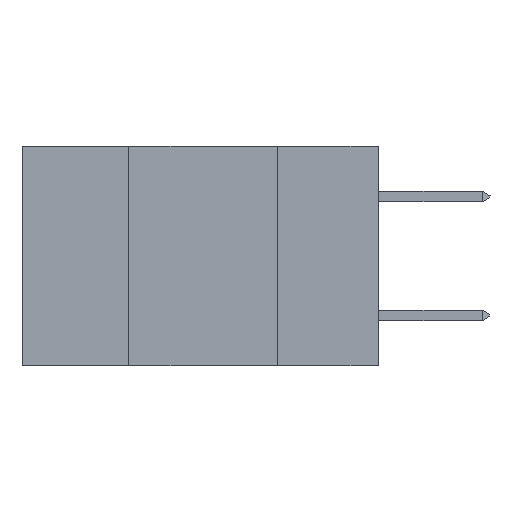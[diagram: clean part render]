
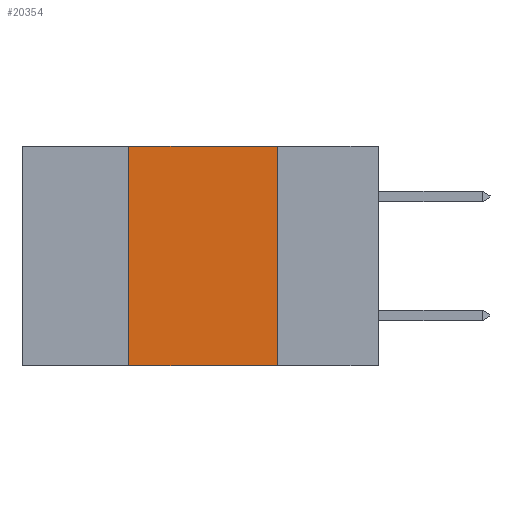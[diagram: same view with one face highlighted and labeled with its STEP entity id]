
A CAD part, left-side view. The second image highlights one B-rep face of the part: STEP entity #20354.
In plain terms, the highlighted planar face has unit normal (-1, 0, 0).
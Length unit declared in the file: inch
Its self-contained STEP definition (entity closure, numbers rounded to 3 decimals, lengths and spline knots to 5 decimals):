
#238 = LINE ( 'NONE', #11202, #19931 ) ;
#572 = VERTEX_POINT ( 'NONE', #11583 ) ;
#872 = EDGE_CURVE ( 'NONE', #572, #17587, #2116, .T. ) ;
#2116 = LINE ( 'NONE', #15072, #17756 ) ;
#3079 = DIRECTION ( 'NONE',  ( 0., 0., -1. ) ) ;
#4374 = DIRECTION ( 'NONE',  ( 0., -1., 0. ) ) ;
#5591 = CARTESIAN_POINT ( 'NONE',  ( 0., 0.6, 0. ) ) ;
#8666 = DIRECTION ( 'NONE',  ( 0., 0., -1. ) ) ;
#9419 = FACE_OUTER_BOUND ( 'NONE', #26075, .T. ) ;
#10312 = CARTESIAN_POINT ( 'NONE',  ( 0., 0.42, -0.37 ) ) ;
#10592 = CARTESIAN_POINT ( 'NONE',  ( 0., 0.17, 0. ) ) ;
#11069 = EDGE_CURVE ( 'NONE', #572, #26701, #14545, .T. ) ;
#11202 = CARTESIAN_POINT ( 'NONE',  ( 0., 0.17, -0.37 ) ) ;
#11583 = CARTESIAN_POINT ( 'NONE',  ( 0., 0.42, -0.37 ) ) ;
#12337 = ORIENTED_EDGE ( 'NONE', *, *, #26849, .F. ) ;
#13105 = VECTOR ( 'NONE', #18578, 39.37008 ) ;
#14545 = LINE ( 'NONE', #10312, #20396 ) ;
#15072 = CARTESIAN_POINT ( 'NONE',  ( 0., 0.6, -0.37 ) ) ;
#16021 = LINE ( 'NONE', #5591, #13105 ) ;
#16310 = PLANE ( 'NONE',  #19810 ) ;
#16771 = ORIENTED_EDGE ( 'NONE', *, *, #11069, .F. ) ;
#17264 = ORIENTED_EDGE ( 'NONE', *, *, #24300, .F. ) ;
#17587 = VERTEX_POINT ( 'NONE', #24310 ) ;
#17756 = VECTOR ( 'NONE', #4374, 39.37008 ) ;
#18514 = DIRECTION ( 'NONE',  ( 0., 0., 1. ) ) ;
#18578 = DIRECTION ( 'NONE',  ( 0., -1., 0. ) ) ;
#19449 = ORIENTED_EDGE ( 'NONE', *, *, #872, .T. ) ;
#19810 = AXIS2_PLACEMENT_3D ( 'NONE', #24906, #26624, #3079 ) ;
#19931 = VECTOR ( 'NONE', #8666, 39.37008 ) ;
#20354 = ADVANCED_FACE ( 'NONE', ( #9419 ), #16310, .F. ) ;
#20396 = VECTOR ( 'NONE', #18514, 39.37008 ) ;
#23210 = CARTESIAN_POINT ( 'NONE',  ( 0., 0.42, 0. ) ) ;
#24300 = EDGE_CURVE ( 'NONE', #26701, #27079, #16021, .T. ) ;
#24310 = CARTESIAN_POINT ( 'NONE',  ( 0., 0.17, -0.37 ) ) ;
#24906 = CARTESIAN_POINT ( 'NONE',  ( 0., 0.6, 0. ) ) ;
#26075 = EDGE_LOOP ( 'NONE', ( #12337, #17264, #16771, #19449 ) ) ;
#26624 = DIRECTION ( 'NONE',  ( 1., 0., 0. ) ) ;
#26701 = VERTEX_POINT ( 'NONE', #23210 ) ;
#26849 = EDGE_CURVE ( 'NONE', #27079, #17587, #238, .T. ) ;
#27079 = VERTEX_POINT ( 'NONE', #10592 ) ;
